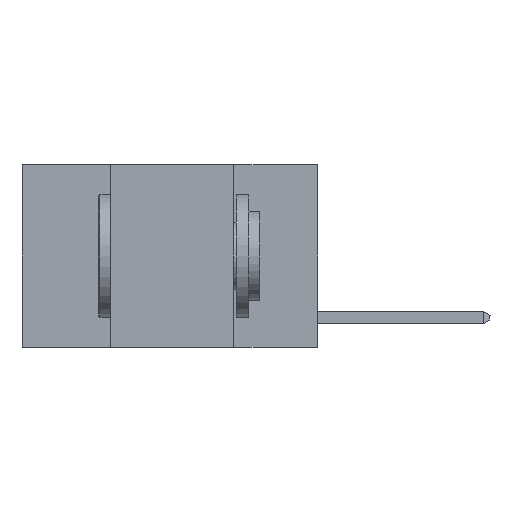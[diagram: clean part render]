
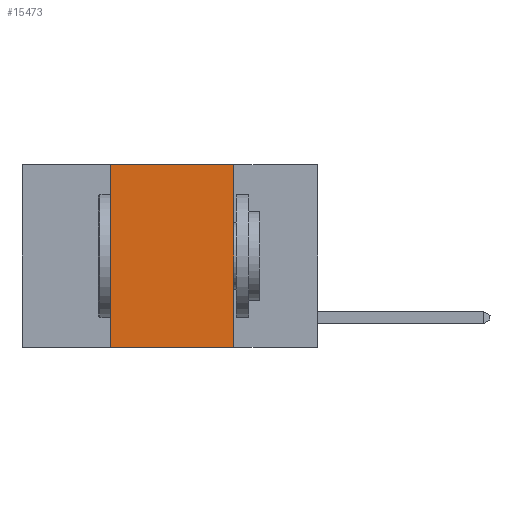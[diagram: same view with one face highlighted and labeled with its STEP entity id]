
A CAD part, left-side view. The second image highlights one B-rep face of the part: STEP entity #15473.
In plain terms, the highlighted planar face has unit normal (-1, 0, 0).
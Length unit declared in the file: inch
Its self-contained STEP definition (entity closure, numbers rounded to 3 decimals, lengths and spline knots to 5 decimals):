
#493 = VERTEX_POINT ( 'NONE', #8597 ) ;
#1453 = EDGE_CURVE ( 'NONE', #17829, #17691, #2013, .T. ) ;
#2013 = LINE ( 'NONE', #18353, #17055 ) ;
#2061 = VECTOR ( 'NONE', #5378, 39.37008 ) ;
#2886 = DIRECTION ( 'NONE',  ( 0., 0., -1. ) ) ;
#3575 = VECTOR ( 'NONE', #2886, 39.37008 ) ;
#4537 = DIRECTION ( 'NONE',  ( 1., 0., 0. ) ) ;
#4688 = CARTESIAN_POINT ( 'NONE',  ( 0., 0.42, -0.37 ) ) ;
#4704 = EDGE_CURVE ( 'NONE', #17829, #20989, #16170, .T. ) ;
#5378 = DIRECTION ( 'NONE',  ( 0., 0., 1. ) ) ;
#6189 = CARTESIAN_POINT ( 'NONE',  ( 0., 0.6, 0. ) ) ;
#8361 = AXIS2_PLACEMENT_3D ( 'NONE', #9962, #4537, #15088 ) ;
#8597 = CARTESIAN_POINT ( 'NONE',  ( 0., 0.17, 0. ) ) ;
#8848 = ORIENTED_EDGE ( 'NONE', *, *, #19474, .F. ) ;
#9962 = CARTESIAN_POINT ( 'NONE',  ( 0., 0.6, 0. ) ) ;
#11650 = CARTESIAN_POINT ( 'NONE',  ( 0., 0.17, 0. ) ) ;
#14259 = ORIENTED_EDGE ( 'NONE', *, *, #19925, .F. ) ;
#14433 = VECTOR ( 'NONE', #15184, 39.37008 ) ;
#15088 = DIRECTION ( 'NONE',  ( 0., 0., -1. ) ) ;
#15184 = DIRECTION ( 'NONE',  ( 0., -1., 0. ) ) ;
#15473 = ADVANCED_FACE ( 'NONE', ( #17334 ), #20532, .F. ) ;
#16170 = LINE ( 'NONE', #17940, #2061 ) ;
#17055 = VECTOR ( 'NONE', #21924, 39.37008 ) ;
#17334 = FACE_OUTER_BOUND ( 'NONE', #22681, .T. ) ;
#17691 = VERTEX_POINT ( 'NONE', #22026 ) ;
#17829 = VERTEX_POINT ( 'NONE', #4688 ) ;
#17839 = ORIENTED_EDGE ( 'NONE', *, *, #1453, .T. ) ;
#17940 = CARTESIAN_POINT ( 'NONE',  ( 0., 0.42, 0. ) ) ;
#18353 = CARTESIAN_POINT ( 'NONE',  ( 0., 0.6, -0.37 ) ) ;
#19474 = EDGE_CURVE ( 'NONE', #493, #17691, #20787, .T. ) ;
#19925 = EDGE_CURVE ( 'NONE', #20989, #493, #20410, .T. ) ;
#20410 = LINE ( 'NONE', #6189, #14433 ) ;
#20532 = PLANE ( 'NONE',  #8361 ) ;
#20787 = LINE ( 'NONE', #11650, #3575 ) ;
#20825 = CARTESIAN_POINT ( 'NONE',  ( 0., 0.42, 0. ) ) ;
#20989 = VERTEX_POINT ( 'NONE', #20825 ) ;
#21924 = DIRECTION ( 'NONE',  ( 0., -1., 0. ) ) ;
#22026 = CARTESIAN_POINT ( 'NONE',  ( 0., 0.17, -0.37 ) ) ;
#22681 = EDGE_LOOP ( 'NONE', ( #8848, #14259, #22911, #17839 ) ) ;
#22911 = ORIENTED_EDGE ( 'NONE', *, *, #4704, .F. ) ;
